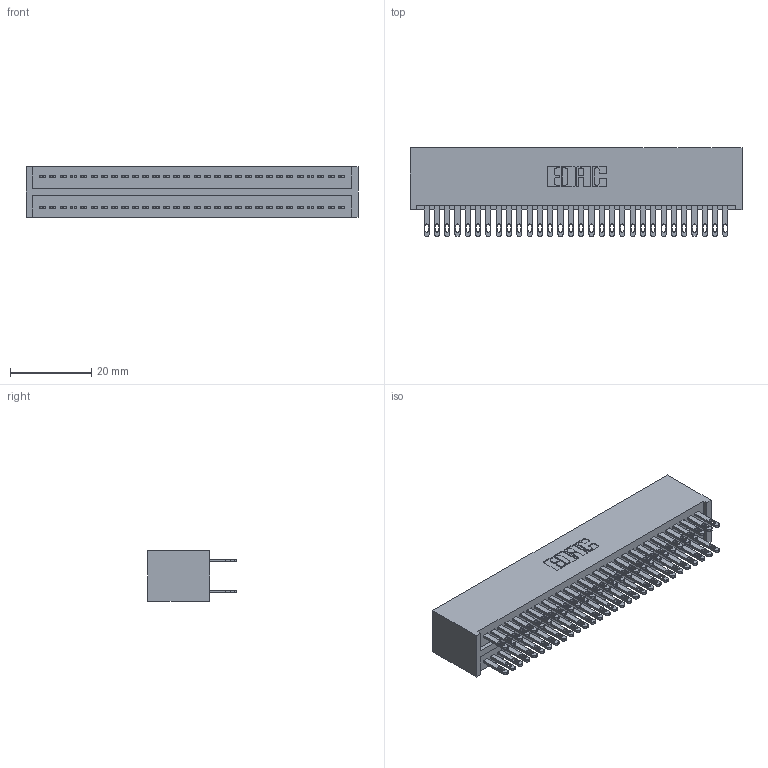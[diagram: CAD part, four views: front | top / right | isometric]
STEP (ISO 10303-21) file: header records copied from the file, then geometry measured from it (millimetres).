
FILE_DESCRIPTION (( 'STEP AP203' ), '1' );
FILE_NAME ('325-060-500-201.STEP', '2020-02-25T02:24:55', ( '' ), ( '' ), 'SwSTEP 2.0', 'SolidWorks 2016', '' );
FILE_SCHEMA (( 'CONFIG_CONTROL_DESIGN' ));
Length unit declared in the file: inch
Products named in the file (3): 325-060-500-201; 325-292-001_325-293-100; 325 Part_Lugless
Assembly tree (61 placements, depth 2):
  325-060-500-201
    325 Part_Lugless
    325-292-001_325-293-100  x60
Bounding box: 81.84 x 21.84 x 12.45 mm (x, y, z)
Volume: 11246.9 mm3; surface area: 14616.7 mm2
Topology: 61 solids, 61 shells, 2986 faces, 9107 edges, 6070 vertices
Faces by surface type: plane 1866, cylinder 1120
Entity records: 20505 total; most frequent: CARTESIAN_POINT 3410, ORIENTED_EDGE 3346, DIRECTION 2929, EDGE_CURVE 1673, VECTOR 1549, LINE 1549, VERTEX_POINT 1114, AXIS2_PLACEMENT_3D 690
